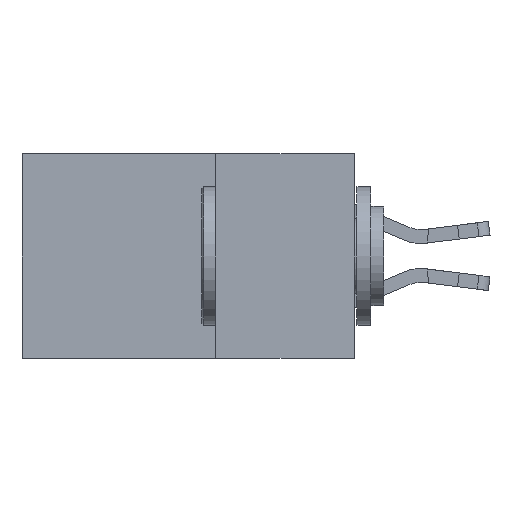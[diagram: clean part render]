
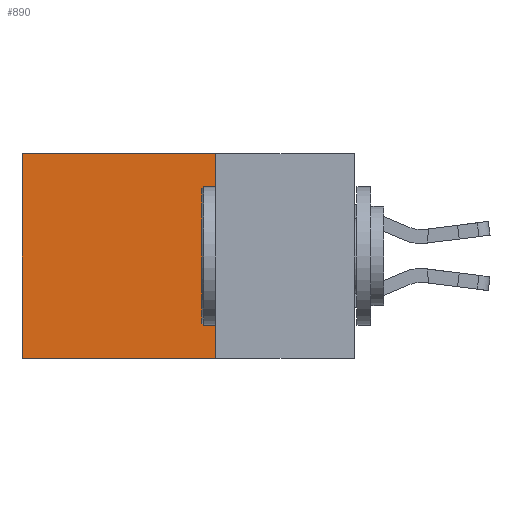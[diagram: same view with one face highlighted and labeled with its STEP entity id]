
A CAD part, left-side view. The second image highlights one B-rep face of the part: STEP entity #890.
In plain terms, the highlighted planar face has unit normal (-1, 0, 0).
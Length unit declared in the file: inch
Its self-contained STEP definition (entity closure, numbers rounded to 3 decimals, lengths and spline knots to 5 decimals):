
#61 = CARTESIAN_POINT ( 'NONE',  ( 0.2615, 0.25, -0.37 ) ) ;
#382 = CARTESIAN_POINT ( 'NONE',  ( 0.2615, 0.25, 0. ) ) ;
#890 = ADVANCED_FACE ( 'NONE', ( #2881 ), #9791, .F. ) ;
#1470 = ORIENTED_EDGE ( 'NONE', *, *, #2130, .T. ) ;
#1720 = DIRECTION ( 'NONE',  ( 0., 0., -1. ) ) ;
#2130 = EDGE_CURVE ( 'NONE', #9329, #2714, #9883, .T. ) ;
#2206 = DIRECTION ( 'NONE',  ( 0., 1., 0. ) ) ;
#2714 = VERTEX_POINT ( 'NONE', #6357 ) ;
#2881 = FACE_OUTER_BOUND ( 'NONE', #9566, .T. ) ;
#3113 = EDGE_CURVE ( 'NONE', #4313, #2714, #6257, .T. ) ;
#3427 = DIRECTION ( 'NONE',  ( 0., 1., 0. ) ) ;
#3674 = CARTESIAN_POINT ( 'NONE',  ( 0.2615, 0.25, 0. ) ) ;
#4281 = DIRECTION ( 'NONE',  ( 0., 0., -1. ) ) ;
#4313 = VERTEX_POINT ( 'NONE', #15778 ) ;
#4838 = CARTESIAN_POINT ( 'NONE',  ( 0.2615, 0.6, 0. ) ) ;
#5533 = LINE ( 'NONE', #61, #6931 ) ;
#5578 = VECTOR ( 'NONE', #1720, 39.37008 ) ;
#5903 = VECTOR ( 'NONE', #2206, 39.37008 ) ;
#6257 = LINE ( 'NONE', #10639, #5903 ) ;
#6357 = CARTESIAN_POINT ( 'NONE',  ( 0.2615, 0.6, -0.37 ) ) ;
#6702 = EDGE_CURVE ( 'NONE', #16642, #4313, #5533, .T. ) ;
#6931 = VECTOR ( 'NONE', #4281, 39.37008 ) ;
#6977 = ORIENTED_EDGE ( 'NONE', *, *, #6702, .F. ) ;
#8541 = CARTESIAN_POINT ( 'NONE',  ( 0.2615, 0.25, -0.37 ) ) ;
#8626 = DIRECTION ( 'NONE',  ( 1., 0., 0. ) ) ;
#8947 = EDGE_CURVE ( 'NONE', #16642, #9329, #10257, .T. ) ;
#9329 = VERTEX_POINT ( 'NONE', #4838 ) ;
#9566 = EDGE_LOOP ( 'NONE', ( #1470, #10314, #6977, #16241 ) ) ;
#9791 = PLANE ( 'NONE',  #11248 ) ;
#9883 = LINE ( 'NONE', #15178, #5578 ) ;
#10257 = LINE ( 'NONE', #382, #12229 ) ;
#10314 = ORIENTED_EDGE ( 'NONE', *, *, #3113, .F. ) ;
#10639 = CARTESIAN_POINT ( 'NONE',  ( 0.2615, 0.25, -0.37 ) ) ;
#11248 = AXIS2_PLACEMENT_3D ( 'NONE', #8541, #8626, #16701 ) ;
#12229 = VECTOR ( 'NONE', #3427, 39.37008 ) ;
#15178 = CARTESIAN_POINT ( 'NONE',  ( 0.2615, 0.6, -0.37 ) ) ;
#15778 = CARTESIAN_POINT ( 'NONE',  ( 0.2615, 0.25, -0.37 ) ) ;
#16241 = ORIENTED_EDGE ( 'NONE', *, *, #8947, .T. ) ;
#16642 = VERTEX_POINT ( 'NONE', #3674 ) ;
#16701 = DIRECTION ( 'NONE',  ( 0., 0., -1. ) ) ;
